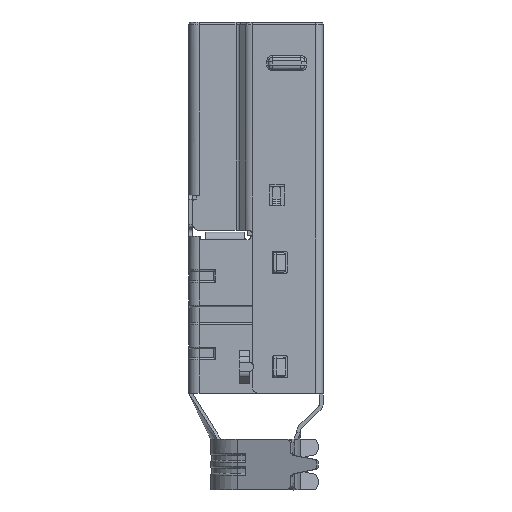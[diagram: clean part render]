
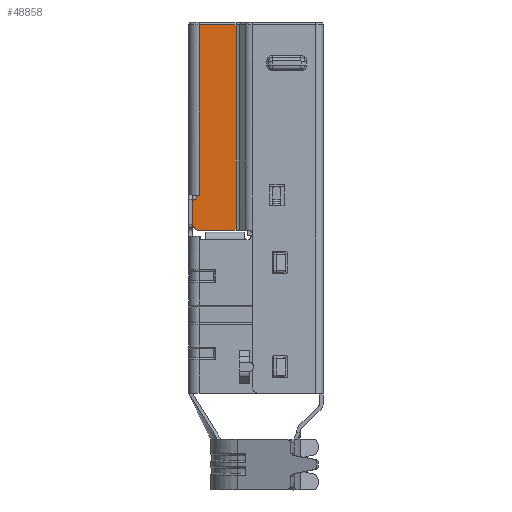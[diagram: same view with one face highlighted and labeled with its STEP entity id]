
A CAD part, left-side view. The second image highlights one B-rep face of the part: STEP entity #48858.
In plain terms, the highlighted planar face has unit normal (-1, 0, 0).
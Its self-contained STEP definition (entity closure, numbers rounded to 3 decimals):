
#826 = VERTEX_POINT ( 'NONE', #8517 ) ;
#1236 = EDGE_CURVE ( 'NONE', #12822, #5723, #47062, .T. ) ;
#1442 = ORIENTED_EDGE ( 'NONE', *, *, #19407, .T. ) ;
#1775 = CARTESIAN_POINT ( 'NONE',  ( -3.196, 3.14, -16.15 ) ) ;
#1940 = DIRECTION ( 'NONE',  ( 0., 1., 0. ) ) ;
#2175 = CARTESIAN_POINT ( 'NONE',  ( -3.196, 6.009, -8.175 ) ) ;
#2272 = VERTEX_POINT ( 'NONE', #35045 ) ;
#2485 = DIRECTION ( 'NONE',  ( 0., 1., 0. ) ) ;
#2936 = DIRECTION ( 'NONE',  ( 0., 0., 1. ) ) ;
#4010 = CIRCLE ( 'NONE', #37650, 0.2 ) ;
#4764 = DIRECTION ( 'NONE',  ( 0., 0., -1. ) ) ;
#5020 = DIRECTION ( 'NONE',  ( 0., -1., 0. ) ) ;
#5370 = CARTESIAN_POINT ( 'NONE',  ( -3.196, 6.309, -13.95 ) ) ;
#5723 = VERTEX_POINT ( 'NONE', #40814 ) ;
#5750 = DIRECTION ( 'NONE',  ( 0., -1., 0. ) ) ;
#6092 = CIRCLE ( 'NONE', #35719, 0.5 ) ;
#7456 = VECTOR ( 'NONE', #20492, 1000. ) ;
#7703 = VECTOR ( 'NONE', #1940, 1000. ) ;
#7710 = DIRECTION ( 'NONE',  ( 0., 0., 1. ) ) ;
#7781 = CARTESIAN_POINT ( 'NONE',  ( -3.196, 6.009, -15.65 ) ) ;
#7871 = EDGE_CURVE ( 'NONE', #25352, #23132, #19166, .T. ) ;
#8023 = EDGE_CURVE ( 'NONE', #826, #2272, #4010, .T. ) ;
#8517 = CARTESIAN_POINT ( 'NONE',  ( -3.196, 6.309, -13.75 ) ) ;
#9370 = DIRECTION ( 'NONE',  ( 0., 0., -1. ) ) ;
#11495 = LINE ( 'NONE', #15474, #46854 ) ;
#11700 = ORIENTED_EDGE ( 'NONE', *, *, #32326, .F. ) ;
#12822 = VERTEX_POINT ( 'NONE', #19597 ) ;
#13021 = CARTESIAN_POINT ( 'NONE',  ( -3.196, 6.259, -13.75 ) ) ;
#15474 = CARTESIAN_POINT ( 'NONE',  ( -3.196, 6.209, -13.6 ) ) ;
#16030 = LINE ( 'NONE', #46641, #40531 ) ;
#16316 = EDGE_CURVE ( 'NONE', #826, #33132, #16756, .T. ) ;
#16756 = LINE ( 'NONE', #13021, #31142 ) ;
#17751 = CARTESIAN_POINT ( 'NONE',  ( -3.196, 3.073, -16.469 ) ) ;
#18240 = CARTESIAN_POINT ( 'NONE',  ( -3.196, 4.825, -13.45 ) ) ;
#18407 = VECTOR ( 'NONE', #34960, 1000. ) ;
#19166 = LINE ( 'NONE', #30706, #18407 ) ;
#19301 = DIRECTION ( 'NONE',  ( -1., 0., 0. ) ) ;
#19407 = EDGE_CURVE ( 'NONE', #23998, #23132, #6092, .T. ) ;
#19430 = VECTOR ( 'NONE', #5750, 1000. ) ;
#19488 = EDGE_CURVE ( 'NONE', #2272, #23998, #16030, .T. ) ;
#19596 = AXIS2_PLACEMENT_3D ( 'NONE', #17751, #33799, #2485 ) ;
#19597 = CARTESIAN_POINT ( 'NONE',  ( -3.196, 3.14, -0.2 ) ) ;
#20492 = DIRECTION ( 'NONE',  ( 0., 0., -1. ) ) ;
#20893 = DIRECTION ( 'NONE',  ( -1., 0., 0. ) ) ;
#21207 = ORIENTED_EDGE ( 'NONE', *, *, #8023, .T. ) ;
#21501 = FACE_OUTER_BOUND ( 'NONE', #35105, .T. ) ;
#22258 = ORIENTED_EDGE ( 'NONE', *, *, #19488, .T. ) ;
#23132 = VERTEX_POINT ( 'NONE', #30631 ) ;
#23956 = ORIENTED_EDGE ( 'NONE', *, *, #48999, .F. ) ;
#23998 = VERTEX_POINT ( 'NONE', #42788 ) ;
#24467 = LINE ( 'NONE', #2175, #48125 ) ;
#25352 = VERTEX_POINT ( 'NONE', #1775 ) ;
#25397 = ORIENTED_EDGE ( 'NONE', *, *, #7871, .F. ) ;
#25819 = CARTESIAN_POINT ( 'NONE',  ( -3.196, 6.209, -13.45 ) ) ;
#27458 = ORIENTED_EDGE ( 'NONE', *, *, #43918, .F. ) ;
#27612 = VERTEX_POINT ( 'NONE', #25819 ) ;
#29861 = CARTESIAN_POINT ( 'NONE',  ( -3.196, 6.009, -13.45 ) ) ;
#30547 = EDGE_CURVE ( 'NONE', #35737, #5723, #24467, .T. ) ;
#30631 = CARTESIAN_POINT ( 'NONE',  ( -3.196, 6.009, -16.15 ) ) ;
#30706 = CARTESIAN_POINT ( 'NONE',  ( -3.196, 4.825, -16.15 ) ) ;
#31142 = VECTOR ( 'NONE', #5020, 1000. ) ;
#31538 = CARTESIAN_POINT ( 'NONE',  ( -3.196, 3.14, -8.175 ) ) ;
#32326 = EDGE_CURVE ( 'NONE', #27612, #35737, #37319, .T. ) ;
#33132 = VERTEX_POINT ( 'NONE', #40230 ) ;
#33799 = DIRECTION ( 'NONE',  ( 1., 0., 0. ) ) ;
#33970 = ORIENTED_EDGE ( 'NONE', *, *, #30547, .F. ) ;
#34960 = DIRECTION ( 'NONE',  ( 0., 1., 0. ) ) ;
#35045 = CARTESIAN_POINT ( 'NONE',  ( -3.196, 6.509, -13.95 ) ) ;
#35105 = EDGE_LOOP ( 'NONE', ( #27458, #37203, #33970, #11700, #23956, #43263, #21207, #22258, #1442, #25397 ) ) ;
#35719 = AXIS2_PLACEMENT_3D ( 'NONE', #7781, #19301, #38881 ) ;
#35737 = VERTEX_POINT ( 'NONE', #29861 ) ;
#37203 = ORIENTED_EDGE ( 'NONE', *, *, #1236, .T. ) ;
#37319 = LINE ( 'NONE', #18240, #19430 ) ;
#37650 = AXIS2_PLACEMENT_3D ( 'NONE', #5370, #20893, #9370 ) ;
#38881 = DIRECTION ( 'NONE',  ( 0., 0., -1. ) ) ;
#40230 = CARTESIAN_POINT ( 'NONE',  ( -3.196, 6.209, -13.75 ) ) ;
#40531 = VECTOR ( 'NONE', #4764, 1000. ) ;
#40814 = CARTESIAN_POINT ( 'NONE',  ( -3.196, 6.009, -0.2 ) ) ;
#40832 = PLANE ( 'NONE',  #19596 ) ;
#42788 = CARTESIAN_POINT ( 'NONE',  ( -3.196, 6.509, -15.65 ) ) ;
#43070 = LINE ( 'NONE', #31538, #7456 ) ;
#43263 = ORIENTED_EDGE ( 'NONE', *, *, #16316, .F. ) ;
#43918 = EDGE_CURVE ( 'NONE', #12822, #25352, #43070, .T. ) ;
#46641 = CARTESIAN_POINT ( 'NONE',  ( -3.196, 6.509, -14.8 ) ) ;
#46829 = CARTESIAN_POINT ( 'NONE',  ( -3.196, 4.575, -0.2 ) ) ;
#46854 = VECTOR ( 'NONE', #7710, 1000. ) ;
#47062 = LINE ( 'NONE', #46829, #7703 ) ;
#48125 = VECTOR ( 'NONE', #2936, 1000. ) ;
#48858 = ADVANCED_FACE ( 'NONE', ( #21501 ), #40832, .F. ) ;
#48999 = EDGE_CURVE ( 'NONE', #33132, #27612, #11495, .T. ) ;
